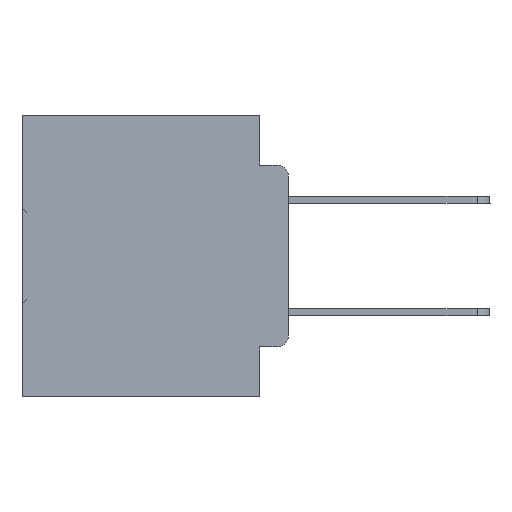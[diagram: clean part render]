
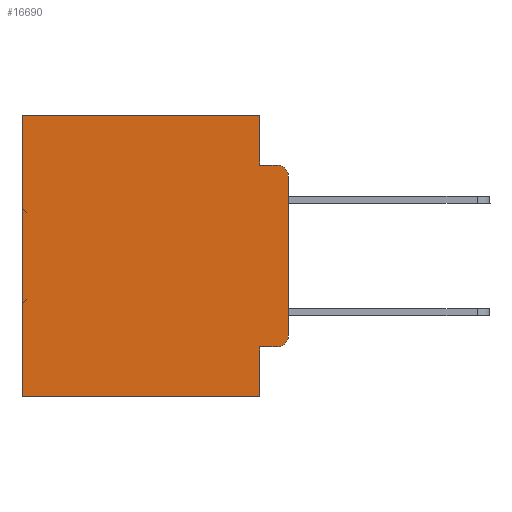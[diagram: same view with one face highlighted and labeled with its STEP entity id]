
A CAD part, left-side view. The second image highlights one B-rep face of the part: STEP entity #16690.
In plain terms, the highlighted planar face has unit normal (-1, 0, 0).
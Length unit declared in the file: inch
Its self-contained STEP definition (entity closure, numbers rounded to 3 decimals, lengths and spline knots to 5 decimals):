
#118 = CARTESIAN_POINT ( 'NONE',  ( 0.298, 0., -0.3915 ) ) ;
#1379 = CARTESIAN_POINT ( 'NONE',  ( 0.298, 0.473, 0. ) ) ;
#1905 = CARTESIAN_POINT ( 'NONE',  ( 0.298, 0.473, -0.5 ) ) ;
#2071 = EDGE_CURVE ( 'NONE', #4003, #4384, #35082, .T. ) ;
#2383 = DIRECTION ( 'NONE',  ( 0., -1., 0. ) ) ;
#2437 = CARTESIAN_POINT ( 'NONE',  ( 0.298, 0., 0. ) ) ;
#3217 = DIRECTION ( 'NONE',  ( 0., 0., -1. ) ) ;
#3319 = DIRECTION ( 'NONE',  ( 0., 0., -1. ) ) ;
#3440 = LINE ( 'NONE', #22139, #32108 ) ;
#4003 = VERTEX_POINT ( 'NONE', #22810 ) ;
#4123 = CARTESIAN_POINT ( 'NONE',  ( 0.298, 0.051, -0.4115 ) ) ;
#4384 = VERTEX_POINT ( 'NONE', #34636 ) ;
#4444 = VERTEX_POINT ( 'NONE', #11552 ) ;
#4936 = ORIENTED_EDGE ( 'NONE', *, *, #10604, .F. ) ;
#4938 = AXIS2_PLACEMENT_3D ( 'NONE', #22397, #24902, #28022 ) ;
#4959 = ORIENTED_EDGE ( 'NONE', *, *, #23825, .T. ) ;
#5752 = ORIENTED_EDGE ( 'NONE', *, *, #13233, .F. ) ;
#5860 = EDGE_CURVE ( 'NONE', #34158, #20839, #10336, .T. ) ;
#5955 = DIRECTION ( 'NONE',  ( -1., 0., 0. ) ) ;
#6664 = VECTOR ( 'NONE', #3217, 39.37008 ) ;
#7439 = VECTOR ( 'NONE', #20059, 39.37008 ) ;
#8023 = LINE ( 'NONE', #21442, #28173 ) ;
#9078 = EDGE_CURVE ( 'NONE', #4003, #10232, #29370, .T. ) ;
#10124 = EDGE_CURVE ( 'NONE', #34158, #4444, #14992, .T. ) ;
#10232 = VERTEX_POINT ( 'NONE', #118 ) ;
#10336 = LINE ( 'NONE', #4123, #12125 ) ;
#10486 = VECTOR ( 'NONE', #12386, 39.37008 ) ;
#10604 = EDGE_CURVE ( 'NONE', #11392, #4384, #36003, .T. ) ;
#10636 = CARTESIAN_POINT ( 'NONE',  ( 0.298, 0.051, -0.0885 ) ) ;
#11392 = VERTEX_POINT ( 'NONE', #16641 ) ;
#11552 = CARTESIAN_POINT ( 'NONE',  ( 0.298, 0.051, -0.5 ) ) ;
#12125 = VECTOR ( 'NONE', #29770, 39.37008 ) ;
#12386 = DIRECTION ( 'NONE',  ( 0., 0., -1. ) ) ;
#12943 = LINE ( 'NONE', #21142, #25492 ) ;
#13109 = EDGE_CURVE ( 'NONE', #23751, #24122, #8023, .T. ) ;
#13110 = FACE_OUTER_BOUND ( 'NONE', #27216, .T. ) ;
#13233 = EDGE_CURVE ( 'NONE', #23751, #11392, #12943, .T. ) ;
#14460 = PLANE ( 'NONE',  #31850 ) ;
#14992 = LINE ( 'NONE', #29765, #10486 ) ;
#16244 = ORIENTED_EDGE ( 'NONE', *, *, #5860, .T. ) ;
#16433 = ORIENTED_EDGE ( 'NONE', *, *, #10124, .F. ) ;
#16641 = CARTESIAN_POINT ( 'NONE',  ( 0.298, 0.051, -0.0885 ) ) ;
#16690 = ADVANCED_FACE ( 'NONE', ( #13110 ), #14460, .F. ) ;
#17572 = DIRECTION ( 'NONE',  ( 1., 0., 0. ) ) ;
#17629 = VECTOR ( 'NONE', #2383, 39.37008 ) ;
#18513 = CARTESIAN_POINT ( 'NONE',  ( 0.298, 0.051, 0. ) ) ;
#20059 = DIRECTION ( 'NONE',  ( 0., 0., -1. ) ) ;
#20206 = CARTESIAN_POINT ( 'NONE',  ( 0.298, 0., 0. ) ) ;
#20340 = CARTESIAN_POINT ( 'NONE',  ( 0.298, 0.473, 0. ) ) ;
#20656 = AXIS2_PLACEMENT_3D ( 'NONE', #31646, #5955, #25976 ) ;
#20721 = CIRCLE ( 'NONE', #4938, 0.02 ) ;
#20839 = VERTEX_POINT ( 'NONE', #35641 ) ;
#21142 = CARTESIAN_POINT ( 'NONE',  ( 0.298, 0.051, 0. ) ) ;
#21442 = CARTESIAN_POINT ( 'NONE',  ( 0.298, 0., 0. ) ) ;
#22139 = CARTESIAN_POINT ( 'NONE',  ( 0.298, 0., -0.5 ) ) ;
#22156 = ORIENTED_EDGE ( 'NONE', *, *, #9078, .F. ) ;
#22397 = CARTESIAN_POINT ( 'NONE',  ( 0.298, 0.02, -0.3915 ) ) ;
#22810 = CARTESIAN_POINT ( 'NONE',  ( 0.298, 0., -0.1085 ) ) ;
#23751 = VERTEX_POINT ( 'NONE', #18513 ) ;
#23825 = EDGE_CURVE ( 'NONE', #20839, #10232, #20721, .T. ) ;
#23947 = DIRECTION ( 'NONE',  ( 0., 1., 0. ) ) ;
#24122 = VERTEX_POINT ( 'NONE', #1379 ) ;
#24287 = DIRECTION ( 'NONE',  ( 0., 0., -1. ) ) ;
#24902 = DIRECTION ( 'NONE',  ( -1., 0., 0. ) ) ;
#25492 = VECTOR ( 'NONE', #24287, 39.37008 ) ;
#25976 = DIRECTION ( 'NONE',  ( 0., 0., -1. ) ) ;
#27216 = EDGE_LOOP ( 'NONE', ( #22156, #27977, #4936, #5752, #31637, #35430, #30300, #16433, #16244, #4959 ) ) ;
#27977 = ORIENTED_EDGE ( 'NONE', *, *, #2071, .T. ) ;
#28009 = DIRECTION ( 'NONE',  ( 0., 1., 0. ) ) ;
#28022 = DIRECTION ( 'NONE',  ( 0., 0., -1. ) ) ;
#28173 = VECTOR ( 'NONE', #23947, 39.37008 ) ;
#29019 = CARTESIAN_POINT ( 'NONE',  ( 0.298, 0.051, -0.4115 ) ) ;
#29370 = LINE ( 'NONE', #2437, #7439 ) ;
#29493 = LINE ( 'NONE', #20340, #6664 ) ;
#29765 = CARTESIAN_POINT ( 'NONE',  ( 0.298, 0.051, 0. ) ) ;
#29770 = DIRECTION ( 'NONE',  ( 0., -1., 0. ) ) ;
#30300 = ORIENTED_EDGE ( 'NONE', *, *, #36755, .F. ) ;
#31637 = ORIENTED_EDGE ( 'NONE', *, *, #13109, .T. ) ;
#31646 = CARTESIAN_POINT ( 'NONE',  ( 0.298, 0.02, -0.1085 ) ) ;
#31850 = AXIS2_PLACEMENT_3D ( 'NONE', #20206, #17572, #3319 ) ;
#32108 = VECTOR ( 'NONE', #28009, 39.37008 ) ;
#33655 = VERTEX_POINT ( 'NONE', #1905 ) ;
#34158 = VERTEX_POINT ( 'NONE', #29019 ) ;
#34636 = CARTESIAN_POINT ( 'NONE',  ( 0.298, 0.02, -0.0885 ) ) ;
#34955 = EDGE_CURVE ( 'NONE', #24122, #33655, #29493, .T. ) ;
#35082 = CIRCLE ( 'NONE', #20656, 0.02 ) ;
#35430 = ORIENTED_EDGE ( 'NONE', *, *, #34955, .T. ) ;
#35641 = CARTESIAN_POINT ( 'NONE',  ( 0.298, 0.02, -0.4115 ) ) ;
#36003 = LINE ( 'NONE', #10636, #17629 ) ;
#36755 = EDGE_CURVE ( 'NONE', #4444, #33655, #3440, .T. ) ;
